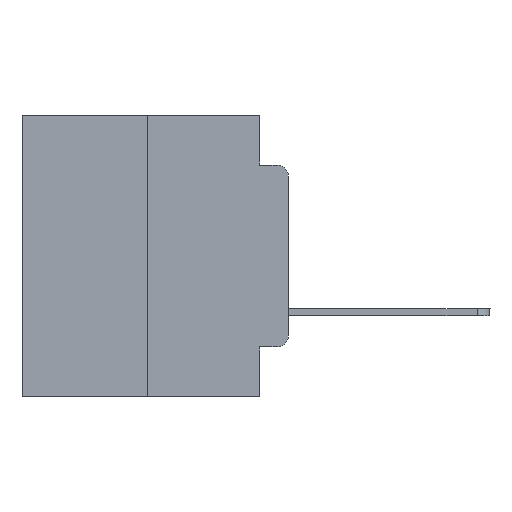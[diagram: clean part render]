
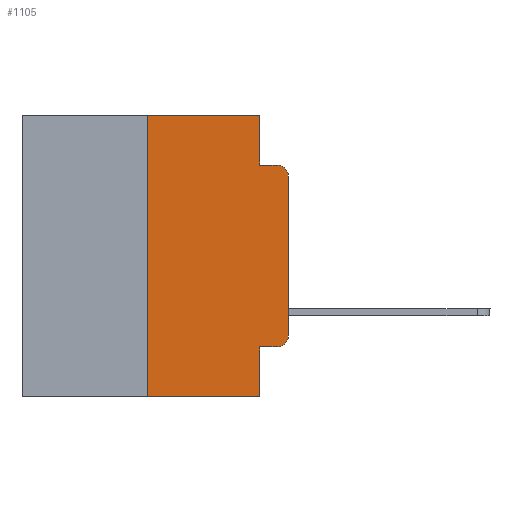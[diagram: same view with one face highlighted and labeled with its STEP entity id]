
A CAD part, left-side view. The second image highlights one B-rep face of the part: STEP entity #1105.
In plain terms, the highlighted planar face has unit normal (-1, 0, 0).
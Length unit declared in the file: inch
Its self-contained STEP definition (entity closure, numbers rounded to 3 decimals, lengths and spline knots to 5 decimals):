
#476 = CIRCLE ( 'NONE', #23231, 0.02 ) ;
#1105 = ADVANCED_FACE ( 'NONE', ( #10861 ), #6244, .F. ) ;
#1854 = VERTEX_POINT ( 'NONE', #18044 ) ;
#2049 = ORIENTED_EDGE ( 'NONE', *, *, #27438, .T. ) ;
#2373 = VERTEX_POINT ( 'NONE', #27054 ) ;
#2852 = CARTESIAN_POINT ( 'NONE',  ( 0., 0.051, 0. ) ) ;
#3001 = DIRECTION ( 'NONE',  ( 0., -1., 0. ) ) ;
#3360 = CARTESIAN_POINT ( 'NONE',  ( 0., 0.473, -0.5 ) ) ;
#4150 = CARTESIAN_POINT ( 'NONE',  ( 0., 0.473, 0. ) ) ;
#4760 = EDGE_CURVE ( 'NONE', #17903, #19204, #476, .T. ) ;
#5406 = EDGE_LOOP ( 'NONE', ( #2049, #21209, #16810, #10785, #7725, #11652, #6443, #24505, #21214, #21918 ) ) ;
#5646 = CARTESIAN_POINT ( 'NONE',  ( 0., 0.051, -0.0885 ) ) ;
#5733 = VECTOR ( 'NONE', #26680, 39.37008 ) ;
#6028 = EDGE_CURVE ( 'NONE', #20849, #25295, #12098, .T. ) ;
#6067 = EDGE_CURVE ( 'NONE', #22038, #24833, #25672, .T. ) ;
#6244 = PLANE ( 'NONE',  #8792 ) ;
#6443 = ORIENTED_EDGE ( 'NONE', *, *, #18025, .T. ) ;
#6603 = CARTESIAN_POINT ( 'NONE',  ( 0., 0., -0.3915 ) ) ;
#6931 = VECTOR ( 'NONE', #27035, 39.37008 ) ;
#7535 = CARTESIAN_POINT ( 'NONE',  ( 0., 0.051, 0. ) ) ;
#7725 = ORIENTED_EDGE ( 'NONE', *, *, #16760, .F. ) ;
#7771 = CARTESIAN_POINT ( 'NONE',  ( 0., 0.25, 0. ) ) ;
#8624 = DIRECTION ( 'NONE',  ( 1., 0., 0. ) ) ;
#8792 = AXIS2_PLACEMENT_3D ( 'NONE', #4150, #8624, #10295 ) ;
#9620 = VECTOR ( 'NONE', #23734, 39.37008 ) ;
#9704 = CARTESIAN_POINT ( 'NONE',  ( 0., 0.051, -0.4115 ) ) ;
#10295 = DIRECTION ( 'NONE',  ( 0., 0., -1. ) ) ;
#10785 = ORIENTED_EDGE ( 'NONE', *, *, #17370, .F. ) ;
#10861 = FACE_OUTER_BOUND ( 'NONE', #5406, .T. ) ;
#11377 = AXIS2_PLACEMENT_3D ( 'NONE', #11680, #27175, #26909 ) ;
#11652 = ORIENTED_EDGE ( 'NONE', *, *, #6028, .F. ) ;
#11680 = CARTESIAN_POINT ( 'NONE',  ( 0., 0.02, -0.1085 ) ) ;
#11939 = CARTESIAN_POINT ( 'NONE',  ( 0., 0.02, -0.3915 ) ) ;
#12098 = LINE ( 'NONE', #7771, #6931 ) ;
#13801 = VERTEX_POINT ( 'NONE', #18019 ) ;
#13904 = VECTOR ( 'NONE', #17643, 39.37008 ) ;
#15101 = CARTESIAN_POINT ( 'NONE',  ( 0., 0.25, 0. ) ) ;
#15790 = CARTESIAN_POINT ( 'NONE',  ( 0., 0.02, -0.4115 ) ) ;
#15812 = EDGE_CURVE ( 'NONE', #2373, #24833, #24663, .T. ) ;
#15815 = EDGE_CURVE ( 'NONE', #13801, #17903, #18502, .T. ) ;
#16760 = EDGE_CURVE ( 'NONE', #25295, #1854, #18675, .T. ) ;
#16810 = ORIENTED_EDGE ( 'NONE', *, *, #15812, .F. ) ;
#17146 = LINE ( 'NONE', #25681, #9620 ) ;
#17370 = EDGE_CURVE ( 'NONE', #1854, #2373, #23939, .T. ) ;
#17643 = DIRECTION ( 'NONE',  ( 0., 0., -1. ) ) ;
#17646 = CARTESIAN_POINT ( 'NONE',  ( 0., 0.02, -0.0885 ) ) ;
#17903 = VERTEX_POINT ( 'NONE', #15790 ) ;
#18019 = CARTESIAN_POINT ( 'NONE',  ( 0., 0.051, -0.4115 ) ) ;
#18025 = EDGE_CURVE ( 'NONE', #20849, #18558, #26279, .T. ) ;
#18044 = CARTESIAN_POINT ( 'NONE',  ( 0., 0.051, 0. ) ) ;
#18136 = DIRECTION ( 'NONE',  ( 0., 0., -1. ) ) ;
#18265 = DIRECTION ( 'NONE',  ( 0., -1., 0. ) ) ;
#18502 = LINE ( 'NONE', #9704, #21952 ) ;
#18558 = VERTEX_POINT ( 'NONE', #24982 ) ;
#18632 = CARTESIAN_POINT ( 'NONE',  ( 0., 0.25, -0.5 ) ) ;
#18675 = LINE ( 'NONE', #22584, #26393 ) ;
#18845 = VECTOR ( 'NONE', #3001, 39.37008 ) ;
#19204 = VERTEX_POINT ( 'NONE', #6603 ) ;
#19839 = EDGE_CURVE ( 'NONE', #13801, #18558, #19842, .T. ) ;
#19842 = LINE ( 'NONE', #7535, #20939 ) ;
#20849 = VERTEX_POINT ( 'NONE', #18632 ) ;
#20939 = VECTOR ( 'NONE', #18136, 39.37008 ) ;
#21209 = ORIENTED_EDGE ( 'NONE', *, *, #6067, .T. ) ;
#21214 = ORIENTED_EDGE ( 'NONE', *, *, #15815, .T. ) ;
#21918 = ORIENTED_EDGE ( 'NONE', *, *, #4760, .T. ) ;
#21952 = VECTOR ( 'NONE', #24371, 39.37008 ) ;
#22038 = VERTEX_POINT ( 'NONE', #26344 ) ;
#22584 = CARTESIAN_POINT ( 'NONE',  ( 0., 0.473, 0. ) ) ;
#23231 = AXIS2_PLACEMENT_3D ( 'NONE', #11939, #26753, #24676 ) ;
#23734 = DIRECTION ( 'NONE',  ( 0., 0., 1. ) ) ;
#23939 = LINE ( 'NONE', #2852, #13904 ) ;
#24371 = DIRECTION ( 'NONE',  ( 0., -1., 0. ) ) ;
#24505 = ORIENTED_EDGE ( 'NONE', *, *, #19839, .F. ) ;
#24663 = LINE ( 'NONE', #5646, #18845 ) ;
#24676 = DIRECTION ( 'NONE',  ( 0., 0., -1. ) ) ;
#24833 = VERTEX_POINT ( 'NONE', #17646 ) ;
#24982 = CARTESIAN_POINT ( 'NONE',  ( 0., 0.051, -0.5 ) ) ;
#25295 = VERTEX_POINT ( 'NONE', #15101 ) ;
#25672 = CIRCLE ( 'NONE', #11377, 0.02 ) ;
#25681 = CARTESIAN_POINT ( 'NONE',  ( 0., 0., 0. ) ) ;
#26279 = LINE ( 'NONE', #3360, #5733 ) ;
#26344 = CARTESIAN_POINT ( 'NONE',  ( 0., 0., -0.1085 ) ) ;
#26393 = VECTOR ( 'NONE', #18265, 39.37008 ) ;
#26680 = DIRECTION ( 'NONE',  ( 0., -1., 0. ) ) ;
#26753 = DIRECTION ( 'NONE',  ( -1., 0., 0. ) ) ;
#26909 = DIRECTION ( 'NONE',  ( 0., 0., -1. ) ) ;
#27035 = DIRECTION ( 'NONE',  ( 0., 0., 1. ) ) ;
#27054 = CARTESIAN_POINT ( 'NONE',  ( 0., 0.051, -0.0885 ) ) ;
#27175 = DIRECTION ( 'NONE',  ( -1., 0., 0. ) ) ;
#27438 = EDGE_CURVE ( 'NONE', #19204, #22038, #17146, .T. ) ;
